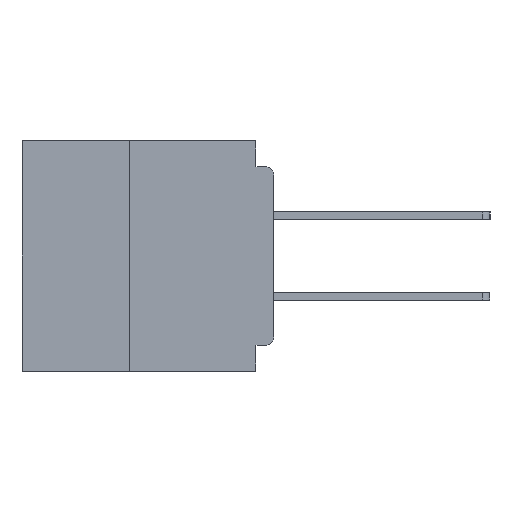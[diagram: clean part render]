
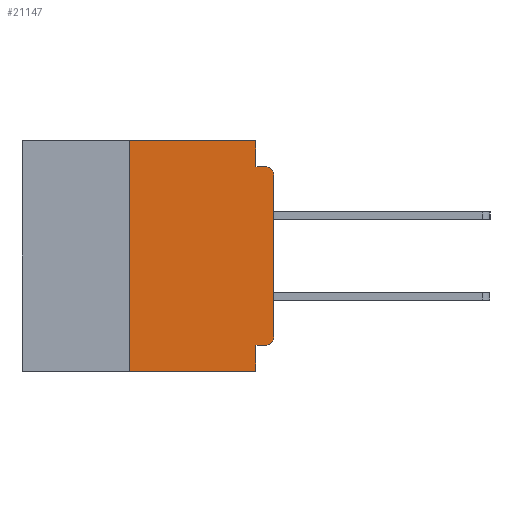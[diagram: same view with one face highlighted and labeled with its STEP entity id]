
A CAD part, left-side view. The second image highlights one B-rep face of the part: STEP entity #21147.
In plain terms, the highlighted planar face has unit normal (-1, 0, 0).
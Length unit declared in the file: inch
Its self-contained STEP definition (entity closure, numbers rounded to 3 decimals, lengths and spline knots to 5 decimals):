
#236 = VERTEX_POINT ( 'NONE', #18060 ) ;
#416 = CARTESIAN_POINT ( 'NONE',  ( 0., 0.031, -0.4 ) ) ;
#472 = FACE_OUTER_BOUND ( 'NONE', #27445, .T. ) ;
#706 = EDGE_CURVE ( 'NONE', #21762, #37881, #36512, .T. ) ;
#990 = CARTESIAN_POINT ( 'NONE',  ( 0., 0.437, -0.4 ) ) ;
#1025 = DIRECTION ( 'NONE',  ( 1., 0., 0. ) ) ;
#1481 = CARTESIAN_POINT ( 'NONE',  ( 0., 0., -0.06 ) ) ;
#2254 = LINE ( 'NONE', #8269, #32750 ) ;
#2915 = VERTEX_POINT ( 'NONE', #16229 ) ;
#3351 = DIRECTION ( 'NONE',  ( 0., -1., 0. ) ) ;
#3801 = VECTOR ( 'NONE', #18392, 39.37008 ) ;
#4186 = DIRECTION ( 'NONE',  ( -1., 0., 0. ) ) ;
#4376 = AXIS2_PLACEMENT_3D ( 'NONE', #9936, #1025, #21832 ) ;
#4970 = CARTESIAN_POINT ( 'NONE',  ( 0., 0.25, -0.4 ) ) ;
#5926 = EDGE_CURVE ( 'NONE', #31475, #17380, #28722, .T. ) ;
#8107 = CARTESIAN_POINT ( 'NONE',  ( 0., 0., -0.34 ) ) ;
#8269 = CARTESIAN_POINT ( 'NONE',  ( 0., 0., 0. ) ) ;
#9031 = AXIS2_PLACEMENT_3D ( 'NONE', #10832, #31412, #13848 ) ;
#9113 = VECTOR ( 'NONE', #16327, 39.37008 ) ;
#9648 = ORIENTED_EDGE ( 'NONE', *, *, #706, .T. ) ;
#9652 = CARTESIAN_POINT ( 'NONE',  ( 0., 0.031, -0.045 ) ) ;
#9842 = LINE ( 'NONE', #4970, #10813 ) ;
#9936 = CARTESIAN_POINT ( 'NONE',  ( 0., 0.437, 0. ) ) ;
#10667 = VECTOR ( 'NONE', #34144, 39.37008 ) ;
#10813 = VECTOR ( 'NONE', #22729, 39.37008 ) ;
#10832 = CARTESIAN_POINT ( 'NONE',  ( 0., 0.015, -0.34 ) ) ;
#11288 = CARTESIAN_POINT ( 'NONE',  ( 0., 0.25, 0. ) ) ;
#11570 = ORIENTED_EDGE ( 'NONE', *, *, #11965, .T. ) ;
#11577 = ORIENTED_EDGE ( 'NONE', *, *, #19704, .F. ) ;
#11965 = EDGE_CURVE ( 'NONE', #33289, #20087, #2254, .T. ) ;
#13295 = VECTOR ( 'NONE', #37807, 39.37008 ) ;
#13848 = DIRECTION ( 'NONE',  ( 0., 0., -1. ) ) ;
#14000 = ORIENTED_EDGE ( 'NONE', *, *, #23064, .F. ) ;
#14232 = LINE ( 'NONE', #35030, #13295 ) ;
#14401 = VERTEX_POINT ( 'NONE', #11288 ) ;
#14866 = EDGE_CURVE ( 'NONE', #2915, #37881, #23913, .T. ) ;
#14984 = EDGE_CURVE ( 'NONE', #23852, #33289, #35667, .T. ) ;
#16229 = CARTESIAN_POINT ( 'NONE',  ( 0., 0.031, -0.355 ) ) ;
#16235 = ORIENTED_EDGE ( 'NONE', *, *, #14984, .T. ) ;
#16327 = DIRECTION ( 'NONE',  ( 0., 0., -1. ) ) ;
#17380 = VERTEX_POINT ( 'NONE', #23909 ) ;
#18060 = CARTESIAN_POINT ( 'NONE',  ( 0., 0.031, 0. ) ) ;
#18392 = DIRECTION ( 'NONE',  ( 0., 1., 0. ) ) ;
#18907 = PLANE ( 'NONE',  #4376 ) ;
#19704 = EDGE_CURVE ( 'NONE', #236, #31475, #14232, .T. ) ;
#20087 = VERTEX_POINT ( 'NONE', #1481 ) ;
#21144 = VECTOR ( 'NONE', #33829, 39.37008 ) ;
#21147 = ADVANCED_FACE ( 'NONE', ( #472 ), #18907, .F. ) ;
#21354 = EDGE_CURVE ( 'NONE', #21762, #14401, #9842, .T. ) ;
#21471 = ORIENTED_EDGE ( 'NONE', *, *, #21809, .T. ) ;
#21762 = VERTEX_POINT ( 'NONE', #36156 ) ;
#21809 = EDGE_CURVE ( 'NONE', #20087, #17380, #23680, .T. ) ;
#21832 = DIRECTION ( 'NONE',  ( 0., 0., -1. ) ) ;
#21982 = CARTESIAN_POINT ( 'NONE',  ( 0., 0.015, -0.06 ) ) ;
#22729 = DIRECTION ( 'NONE',  ( 0., 0., 1. ) ) ;
#23064 = EDGE_CURVE ( 'NONE', #14401, #236, #34049, .T. ) ;
#23680 = CIRCLE ( 'NONE', #31397, 0.015 ) ;
#23852 = VERTEX_POINT ( 'NONE', #34840 ) ;
#23909 = CARTESIAN_POINT ( 'NONE',  ( 0., 0.015, -0.045 ) ) ;
#23913 = LINE ( 'NONE', #36581, #9113 ) ;
#24928 = DIRECTION ( 'NONE',  ( 0., 0., -1. ) ) ;
#25490 = ORIENTED_EDGE ( 'NONE', *, *, #29797, .F. ) ;
#25841 = ORIENTED_EDGE ( 'NONE', *, *, #5926, .F. ) ;
#26175 = ORIENTED_EDGE ( 'NONE', *, *, #21354, .F. ) ;
#27087 = CARTESIAN_POINT ( 'NONE',  ( 0., 0., -0.045 ) ) ;
#27090 = CARTESIAN_POINT ( 'NONE',  ( 0., 0., -0.355 ) ) ;
#27445 = EDGE_LOOP ( 'NONE', ( #11570, #21471, #25841, #11577, #14000, #26175, #9648, #28402, #25490, #16235 ) ) ;
#27781 = VECTOR ( 'NONE', #3351, 39.37008 ) ;
#28402 = ORIENTED_EDGE ( 'NONE', *, *, #14866, .F. ) ;
#28722 = LINE ( 'NONE', #27087, #27781 ) ;
#29797 = EDGE_CURVE ( 'NONE', #23852, #2915, #35992, .T. ) ;
#31274 = CARTESIAN_POINT ( 'NONE',  ( 0., 0.437, 0. ) ) ;
#31397 = AXIS2_PLACEMENT_3D ( 'NONE', #21982, #4186, #24928 ) ;
#31412 = DIRECTION ( 'NONE',  ( -1., 0., 0. ) ) ;
#31475 = VERTEX_POINT ( 'NONE', #9652 ) ;
#32750 = VECTOR ( 'NONE', #37493, 39.37008 ) ;
#33289 = VERTEX_POINT ( 'NONE', #8107 ) ;
#33829 = DIRECTION ( 'NONE',  ( 0., -1., 0. ) ) ;
#34049 = LINE ( 'NONE', #31274, #10667 ) ;
#34144 = DIRECTION ( 'NONE',  ( 0., -1., 0. ) ) ;
#34840 = CARTESIAN_POINT ( 'NONE',  ( 0., 0.015, -0.355 ) ) ;
#35030 = CARTESIAN_POINT ( 'NONE',  ( 0., 0.031, 0. ) ) ;
#35667 = CIRCLE ( 'NONE', #9031, 0.015 ) ;
#35992 = LINE ( 'NONE', #27090, #3801 ) ;
#36156 = CARTESIAN_POINT ( 'NONE',  ( 0., 0.25, -0.4 ) ) ;
#36512 = LINE ( 'NONE', #990, #21144 ) ;
#36581 = CARTESIAN_POINT ( 'NONE',  ( 0., 0.031, -0.4 ) ) ;
#37493 = DIRECTION ( 'NONE',  ( 0., 0., 1. ) ) ;
#37807 = DIRECTION ( 'NONE',  ( 0., 0., -1. ) ) ;
#37881 = VERTEX_POINT ( 'NONE', #416 ) ;
